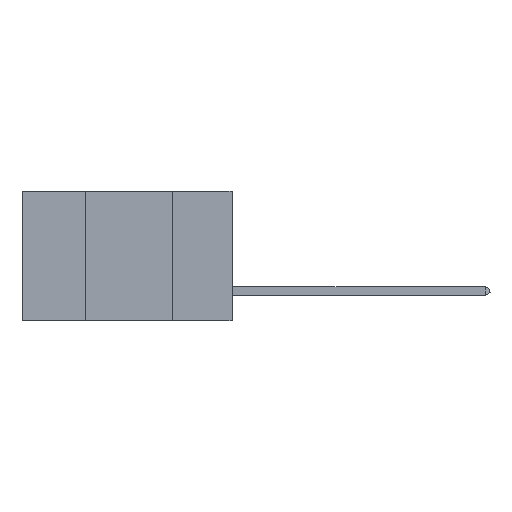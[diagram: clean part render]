
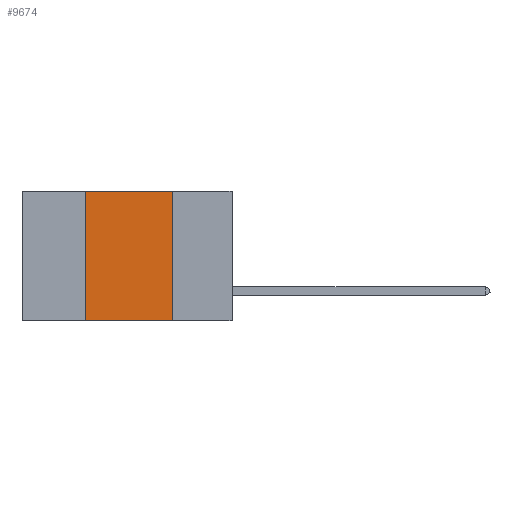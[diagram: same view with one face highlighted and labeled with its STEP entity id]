
A CAD part, left-side view. The second image highlights one B-rep face of the part: STEP entity #9674.
In plain terms, the highlighted planar face has unit normal (-1, 0, 0).
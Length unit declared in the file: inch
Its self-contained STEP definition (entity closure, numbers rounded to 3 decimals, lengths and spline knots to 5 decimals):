
#848 = VERTEX_POINT ( 'NONE', #4984 ) ;
#1335 = DIRECTION ( 'NONE',  ( 0., 0., 1. ) ) ;
#1873 = VECTOR ( 'NONE', #1335, 39.37008 ) ;
#1937 = DIRECTION ( 'NONE',  ( 0., 0., -1. ) ) ;
#2393 = ORIENTED_EDGE ( 'NONE', *, *, #13535, .F. ) ;
#2752 = VECTOR ( 'NONE', #4817, 39.37008 ) ;
#3459 = VERTEX_POINT ( 'NONE', #10870 ) ;
#3595 = VERTEX_POINT ( 'NONE', #8665 ) ;
#3756 = CARTESIAN_POINT ( 'NONE',  ( 0., 0.17, 0. ) ) ;
#4817 = DIRECTION ( 'NONE',  ( 0., 0., -1. ) ) ;
#4915 = PLANE ( 'NONE',  #5517 ) ;
#4984 = CARTESIAN_POINT ( 'NONE',  ( 0., 0.17, 0. ) ) ;
#5517 = AXIS2_PLACEMENT_3D ( 'NONE', #7204, #6068, #1937 ) ;
#5545 = LINE ( 'NONE', #3756, #2752 ) ;
#6068 = DIRECTION ( 'NONE',  ( 1., 0., 0. ) ) ;
#6225 = LINE ( 'NONE', #6287, #11337 ) ;
#6250 = DIRECTION ( 'NONE',  ( 0., -1., 0. ) ) ;
#6287 = CARTESIAN_POINT ( 'NONE',  ( 0., 0.6, -0.37 ) ) ;
#6556 = VECTOR ( 'NONE', #11439, 39.37008 ) ;
#7085 = VERTEX_POINT ( 'NONE', #13159 ) ;
#7204 = CARTESIAN_POINT ( 'NONE',  ( 0., 0.6, 0. ) ) ;
#8665 = CARTESIAN_POINT ( 'NONE',  ( 0., 0.42, 0. ) ) ;
#8841 = ORIENTED_EDGE ( 'NONE', *, *, #10191, .F. ) ;
#9674 = ADVANCED_FACE ( 'NONE', ( #10217 ), #4915, .F. ) ;
#9987 = LINE ( 'NONE', #11821, #1873 ) ;
#10191 = EDGE_CURVE ( 'NONE', #848, #3459, #5545, .T. ) ;
#10217 = FACE_OUTER_BOUND ( 'NONE', #13524, .T. ) ;
#10364 = CARTESIAN_POINT ( 'NONE',  ( 0., 0.6, 0. ) ) ;
#10830 = ORIENTED_EDGE ( 'NONE', *, *, #11061, .F. ) ;
#10870 = CARTESIAN_POINT ( 'NONE',  ( 0., 0.17, -0.37 ) ) ;
#11061 = EDGE_CURVE ( 'NONE', #3595, #848, #12183, .T. ) ;
#11337 = VECTOR ( 'NONE', #6250, 39.37008 ) ;
#11439 = DIRECTION ( 'NONE',  ( 0., -1., 0. ) ) ;
#11749 = EDGE_CURVE ( 'NONE', #7085, #3459, #6225, .T. ) ;
#11821 = CARTESIAN_POINT ( 'NONE',  ( 0., 0.42, 0. ) ) ;
#12183 = LINE ( 'NONE', #10364, #6556 ) ;
#13159 = CARTESIAN_POINT ( 'NONE',  ( 0., 0.42, -0.37 ) ) ;
#13472 = ORIENTED_EDGE ( 'NONE', *, *, #11749, .T. ) ;
#13524 = EDGE_LOOP ( 'NONE', ( #8841, #10830, #2393, #13472 ) ) ;
#13535 = EDGE_CURVE ( 'NONE', #7085, #3595, #9987, .T. ) ;
